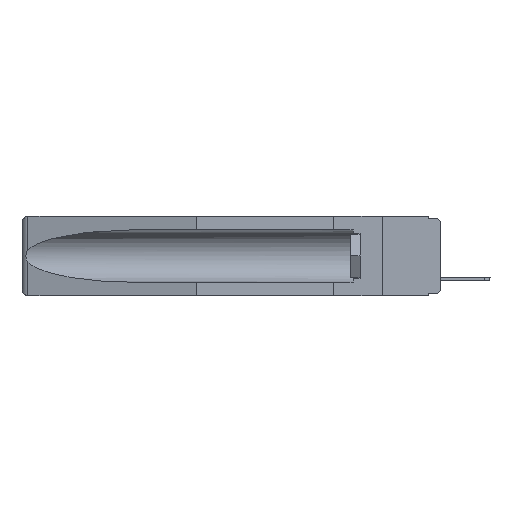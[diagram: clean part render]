
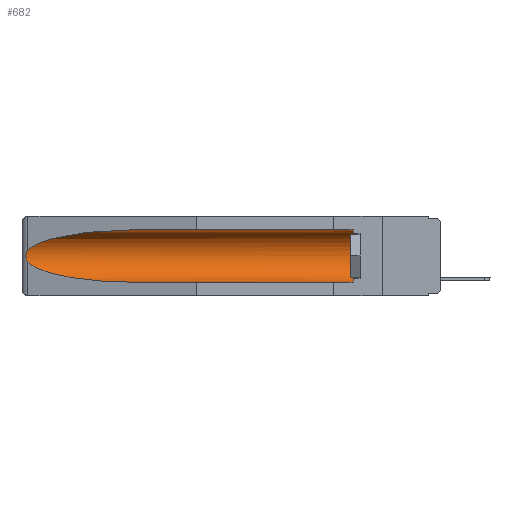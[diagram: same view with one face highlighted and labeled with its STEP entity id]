
A CAD part, left-side view. The second image highlights one B-rep face of the part: STEP entity #682.
In plain terms, the highlighted cylindrical face has radius 2.857 mm (diameter 5.715 mm), a partial arc.
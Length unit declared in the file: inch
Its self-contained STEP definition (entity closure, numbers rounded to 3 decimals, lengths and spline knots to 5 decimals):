
#193 = AXIS2_PLACEMENT_3D ( 'NONE', #4718, #20726, #20794 ) ;
#438 = CARTESIAN_POINT ( 'NONE',  ( 0.26537, 1.52718, -0.19328 ) ) ;
#682 = ADVANCED_FACE ( 'NONE', ( #11043 ), #6299, .F. ) ;
#1576 = CARTESIAN_POINT ( 'NONE',  ( 0.155, 1.07973, -0.059 ) ) ;
#2082 = CARTESIAN_POINT ( 'NONE',  ( 0.155, 0.126, -0.059 ) ) ;
#2821 = CARTESIAN_POINT ( 'NONE',  ( 0.26537, 1.52718, -0.14972 ) ) ;
#3633 = CARTESIAN_POINT ( 'NONE',  ( 0.26537, 1.52718, -0.14972 ) ) ;
#4232 = CARTESIAN_POINT ( 'NONE',  ( 0.155, 0.126, -0.284 ) ) ;
#4718 = CARTESIAN_POINT ( 'NONE',  ( 0.155, -0.30754, -0.1715 ) ) ;
#4883 = CARTESIAN_POINT ( 'NONE',  ( 0.155, 1.07973, -0.059 ) ) ;
#5324 = CARTESIAN_POINT ( 'NONE',  ( 0.26537, 1.52718, -0.19328 ) ) ;
#5379 = CARTESIAN_POINT ( 'NONE',  ( 0.26655, 1.53094, -0.18657 ) ) ;
#5499 = CARTESIAN_POINT ( 'NONE',  ( 0.155, -0.30754, -0.059 ) ) ;
#5662 = CIRCLE ( 'NONE', #18631, 0.1125 ) ;
#6201 = DIRECTION ( 'NONE',  ( 0., 1., 0. ) ) ;
#6299 = CYLINDRICAL_SURFACE ( 'NONE', #193, 0.1125 ) ;
#6455 = VERTEX_POINT ( 'NONE', #1576 ) ;
#6761 = CARTESIAN_POINT ( 'NONE',  ( 0.26654, 1.53092, -0.15636 ) ) ;
#6770 = CARTESIAN_POINT ( 'NONE',  ( 0.26537, 1.52718, -0.19328 ) ) ;
#7077 = VERTEX_POINT ( 'NONE', #7176 ) ;
#7176 = CARTESIAN_POINT ( 'NONE',  ( 0.155, 1.07973, -0.284 ) ) ;
#7348 =( BOUNDED_CURVE ( )  B_SPLINE_CURVE ( 3, ( #4883, #11242, #14405, #12722 ),
 .UNSPECIFIED., .F., .F. ) 
 B_SPLINE_CURVE_WITH_KNOTS ( ( 4, 4 ),
 ( 4.71239, 6.08839 ),
 .UNSPECIFIED. ) 
 CURVE ( )  GEOMETRIC_REPRESENTATION_ITEM ( )  RATIONAL_B_SPLINE_CURVE ( ( 1., 0.848, 0.848, 1. ) ) 
 REPRESENTATION_ITEM ( '' )  );
#7467 = DIRECTION ( 'NONE',  ( 0., 1., 0. ) ) ;
#7930 = ORIENTED_EDGE ( 'NONE', *, *, #17983, .F. ) ;
#8382 = CARTESIAN_POINT ( 'NONE',  ( 0.2675, 1.53308, -0.17534 ) ) ;
#8443 = CARTESIAN_POINT ( 'NONE',  ( 0.26597, 1.52961, -0.15275 ) ) ;
#8785 = EDGE_CURVE ( 'NONE', #13030, #7077, #15400, .T. ) ;
#8798 = VECTOR ( 'NONE', #7467, 39.37008 ) ;
#9089 = DIRECTION ( 'NONE',  ( 0., -1., 0. ) ) ;
#9630 = VERTEX_POINT ( 'NONE', #2082 ) ;
#9959 = CARTESIAN_POINT ( 'NONE',  ( 0.2673, 1.53269, -0.17917 ) ) ;
#10285 = ORIENTED_EDGE ( 'NONE', *, *, #19264, .T. ) ;
#11043 = FACE_OUTER_BOUND ( 'NONE', #17048, .T. ) ;
#11205 = EDGE_CURVE ( 'NONE', #9630, #6455, #13026, .T. ) ;
#11242 = CARTESIAN_POINT ( 'NONE',  ( 0.21114, 1.30732, -0.059 ) ) ;
#11929 = CARTESIAN_POINT ( 'NONE',  ( 0.155, 1.07973, -0.284 ) ) ;
#12275 = CARTESIAN_POINT ( 'NONE',  ( 0.155, 0.126, -0.1715 ) ) ;
#12407 = DIRECTION ( 'NONE',  ( 0., 0., 1. ) ) ;
#12500 = VERTEX_POINT ( 'NONE', #4232 ) ;
#12722 = CARTESIAN_POINT ( 'NONE',  ( 0.26537, 1.52718, -0.14972 ) ) ;
#12903 = ORIENTED_EDGE ( 'NONE', *, *, #14728, .T. ) ;
#13026 = LINE ( 'NONE', #5499, #8798 ) ;
#13030 = VERTEX_POINT ( 'NONE', #6770 ) ;
#13239 = CARTESIAN_POINT ( 'NONE',  ( 0.2675, 1.53308, -0.16763 ) ) ;
#13322 = VERTEX_POINT ( 'NONE', #2821 ) ;
#14026 = ORIENTED_EDGE ( 'NONE', *, *, #15725, .T. ) ;
#14405 = CARTESIAN_POINT ( 'NONE',  ( 0.25451, 1.48313, -0.09465 ) ) ;
#14728 = EDGE_CURVE ( 'NONE', #12500, #9630, #5662, .T. ) ;
#14790 = CARTESIAN_POINT ( 'NONE',  ( 0.26597, 1.5296, -0.19026 ) ) ;
#15400 =( BOUNDED_CURVE ( )  B_SPLINE_CURVE ( 3, ( #5324, #18422, #18194, #11929 ),
 .UNSPECIFIED., .F., .F. ) 
 B_SPLINE_CURVE_WITH_KNOTS ( ( 4, 4 ),
 ( 0.1948, 1.5708 ),
 .UNSPECIFIED. ) 
 CURVE ( )  GEOMETRIC_REPRESENTATION_ITEM ( )  RATIONAL_B_SPLINE_CURVE ( ( 1., 0.848, 0.848, 1. ) ) 
 REPRESENTATION_ITEM ( '' )  );
#15500 = ORIENTED_EDGE ( 'NONE', *, *, #8785, .T. ) ;
#15651 = B_SPLINE_CURVE_WITH_KNOTS ( 'NONE', 3,
 ( #3633, #8443, #6761, #17977, #13239, #8382, #9959, #5379, #14790, #438 ),
 .UNSPECIFIED., .F., .F.,
 ( 4, 2, 2, 2, 4 ),
 ( 0., 0.00029, 0.00058, 0.00087, 0.00117 ),
 .UNSPECIFIED. ) ;
#15725 = EDGE_CURVE ( 'NONE', #13322, #13030, #15651, .T. ) ;
#15768 = CARTESIAN_POINT ( 'NONE',  ( 0.155, -0.30754, -0.284 ) ) ;
#15912 = LINE ( 'NONE', #15768, #17222 ) ;
#16153 = ORIENTED_EDGE ( 'NONE', *, *, #11205, .T. ) ;
#17048 = EDGE_LOOP ( 'NONE', ( #10285, #14026, #15500, #7930, #12903, #16153 ) ) ;
#17222 = VECTOR ( 'NONE', #6201, 39.37008 ) ;
#17977 = CARTESIAN_POINT ( 'NONE',  ( 0.2673, 1.5327, -0.16383 ) ) ;
#17983 = EDGE_CURVE ( 'NONE', #12500, #7077, #15912, .T. ) ;
#18194 = CARTESIAN_POINT ( 'NONE',  ( 0.21114, 1.30732, -0.284 ) ) ;
#18422 = CARTESIAN_POINT ( 'NONE',  ( 0.25451, 1.48313, -0.24835 ) ) ;
#18631 = AXIS2_PLACEMENT_3D ( 'NONE', #12275, #9089, #12407 ) ;
#19264 = EDGE_CURVE ( 'NONE', #6455, #13322, #7348, .T. ) ;
#20726 = DIRECTION ( 'NONE',  ( 0., 1., 0. ) ) ;
#20794 = DIRECTION ( 'NONE',  ( 0., 0., 1. ) ) ;
